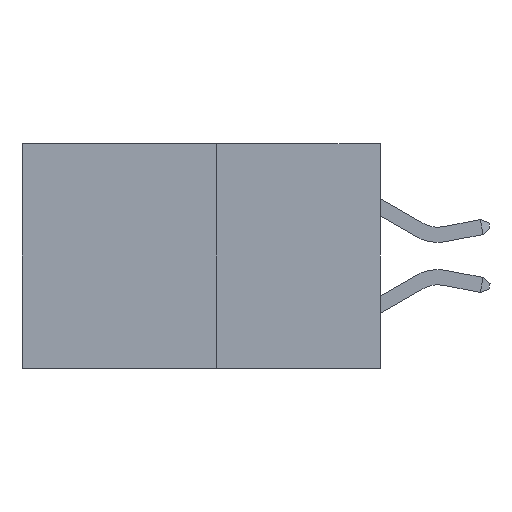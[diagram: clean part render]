
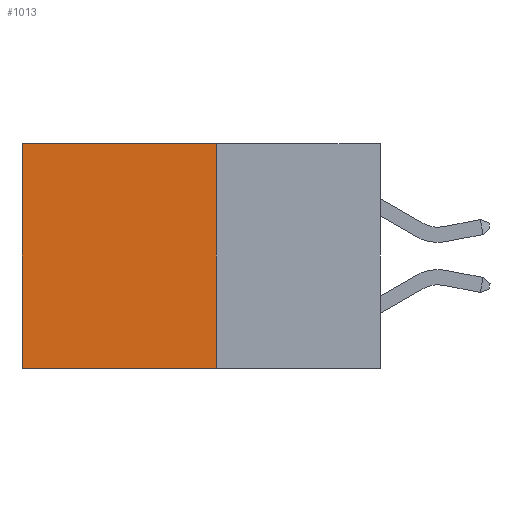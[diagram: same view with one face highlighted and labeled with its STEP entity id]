
A CAD part, left-side view. The second image highlights one B-rep face of the part: STEP entity #1013.
In plain terms, the highlighted planar face has unit normal (-1, 0, 0).
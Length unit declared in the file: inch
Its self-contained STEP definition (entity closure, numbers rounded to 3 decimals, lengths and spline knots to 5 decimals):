
#656 = EDGE_CURVE ( 'NONE', #2058, #4786, #10082, .T. ) ;
#717 = VECTOR ( 'NONE', #8604, 39.37008 ) ;
#1013 = ADVANCED_FACE ( 'NONE', ( #8099 ), #3417, .F. ) ;
#1617 = AXIS2_PLACEMENT_3D ( 'NONE', #9841, #9937, #7284 ) ;
#1811 = VECTOR ( 'NONE', #5072, 39.37008 ) ;
#1959 = VECTOR ( 'NONE', #6835, 39.37008 ) ;
#2058 = VERTEX_POINT ( 'NONE', #7925 ) ;
#2163 = VERTEX_POINT ( 'NONE', #8111 ) ;
#3291 = DIRECTION ( 'NONE',  ( 0., 1., 0. ) ) ;
#3417 = PLANE ( 'NONE',  #1617 ) ;
#4150 = EDGE_CURVE ( 'NONE', #2058, #7356, #9460, .T. ) ;
#4165 = CARTESIAN_POINT ( 'NONE',  ( 0.277, 0.59, 0. ) ) ;
#4339 = EDGE_CURVE ( 'NONE', #7356, #2163, #6276, .T. ) ;
#4786 = VERTEX_POINT ( 'NONE', #7998 ) ;
#4898 = CARTESIAN_POINT ( 'NONE',  ( 0.277, 0.27, -0.37 ) ) ;
#5072 = DIRECTION ( 'NONE',  ( 0., 0., -1. ) ) ;
#5199 = CARTESIAN_POINT ( 'NONE',  ( 0.277, 0.27, -0.37 ) ) ;
#5500 = EDGE_CURVE ( 'NONE', #4786, #2163, #7961, .T. ) ;
#5811 = CARTESIAN_POINT ( 'NONE',  ( 0.277, 0.59, -0.37 ) ) ;
#6124 = VECTOR ( 'NONE', #3291, 39.37008 ) ;
#6276 = LINE ( 'NONE', #5811, #1811 ) ;
#6440 = ORIENTED_EDGE ( 'NONE', *, *, #4339, .T. ) ;
#6835 = DIRECTION ( 'NONE',  ( 0., 0., -1. ) ) ;
#7041 = ORIENTED_EDGE ( 'NONE', *, *, #5500, .F. ) ;
#7106 = ORIENTED_EDGE ( 'NONE', *, *, #656, .F. ) ;
#7284 = DIRECTION ( 'NONE',  ( 0., 0., -1. ) ) ;
#7356 = VERTEX_POINT ( 'NONE', #4165 ) ;
#7925 = CARTESIAN_POINT ( 'NONE',  ( 0.277, 0.27, 0. ) ) ;
#7961 = LINE ( 'NONE', #4898, #6124 ) ;
#7998 = CARTESIAN_POINT ( 'NONE',  ( 0.277, 0.27, -0.37 ) ) ;
#8099 = FACE_OUTER_BOUND ( 'NONE', #8379, .T. ) ;
#8111 = CARTESIAN_POINT ( 'NONE',  ( 0.277, 0.59, -0.37 ) ) ;
#8291 = ORIENTED_EDGE ( 'NONE', *, *, #4150, .T. ) ;
#8379 = EDGE_LOOP ( 'NONE', ( #6440, #7041, #7106, #8291 ) ) ;
#8505 = CARTESIAN_POINT ( 'NONE',  ( 0.277, 0.27, 0. ) ) ;
#8604 = DIRECTION ( 'NONE',  ( 0., 1., 0. ) ) ;
#9460 = LINE ( 'NONE', #8505, #717 ) ;
#9841 = CARTESIAN_POINT ( 'NONE',  ( 0.277, 0.27, -0.37 ) ) ;
#9937 = DIRECTION ( 'NONE',  ( 1., 0., 0. ) ) ;
#10082 = LINE ( 'NONE', #5199, #1959 ) ;
